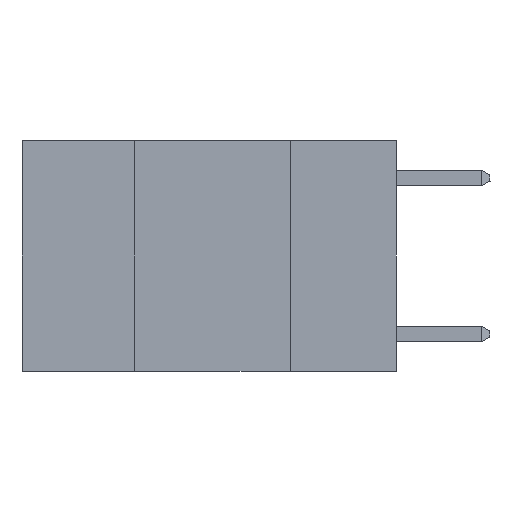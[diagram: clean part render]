
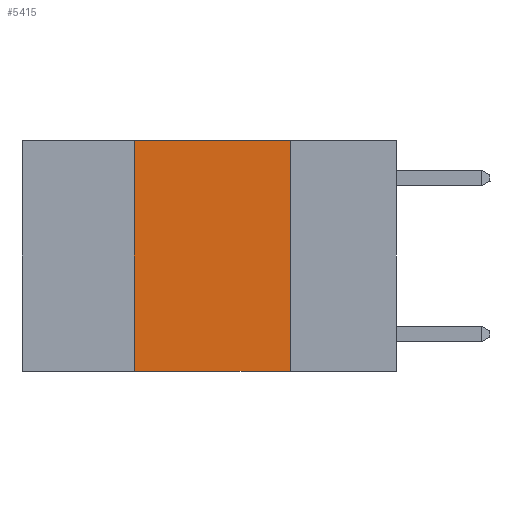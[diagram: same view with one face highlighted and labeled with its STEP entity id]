
A CAD part, left-side view. The second image highlights one B-rep face of the part: STEP entity #5415.
In plain terms, the highlighted planar face has unit normal (-1, 0, 0).
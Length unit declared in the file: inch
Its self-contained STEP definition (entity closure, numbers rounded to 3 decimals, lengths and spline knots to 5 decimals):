
#32 = VERTEX_POINT ( 'NONE', #3492 ) ;
#42 = CARTESIAN_POINT ( 'NONE',  ( 0., 0.17, -0.37 ) ) ;
#235 = VECTOR ( 'NONE', #409, 39.37008 ) ;
#409 = DIRECTION ( 'NONE',  ( 0., -1., 0. ) ) ;
#447 = DIRECTION ( 'NONE',  ( 0., 0., -1. ) ) ;
#834 = CARTESIAN_POINT ( 'NONE',  ( 0., 0.6, 0. ) ) ;
#1045 = VECTOR ( 'NONE', #3212, 39.37008 ) ;
#1571 = DIRECTION ( 'NONE',  ( 0., 0., -1. ) ) ;
#1638 = FACE_OUTER_BOUND ( 'NONE', #7906, .T. ) ;
#1929 = VECTOR ( 'NONE', #447, 39.37008 ) ;
#2073 = EDGE_CURVE ( 'NONE', #32, #7434, #4094, .T. ) ;
#2083 = ORIENTED_EDGE ( 'NONE', *, *, #8897, .T. ) ;
#2264 = AXIS2_PLACEMENT_3D ( 'NONE', #834, #6049, #1571 ) ;
#2320 = VERTEX_POINT ( 'NONE', #5282 ) ;
#2329 = CARTESIAN_POINT ( 'NONE',  ( 0., 0.42, 0. ) ) ;
#2740 = ORIENTED_EDGE ( 'NONE', *, *, #4214, .F. ) ;
#3212 = DIRECTION ( 'NONE',  ( 0., 0., 1. ) ) ;
#3402 = ORIENTED_EDGE ( 'NONE', *, *, #2073, .F. ) ;
#3492 = CARTESIAN_POINT ( 'NONE',  ( 0., 0.17, 0. ) ) ;
#4094 = LINE ( 'NONE', #5994, #1929 ) ;
#4214 = EDGE_CURVE ( 'NONE', #7386, #32, #8233, .T. ) ;
#4279 = CARTESIAN_POINT ( 'NONE',  ( 0., 0.6, 0. ) ) ;
#5282 = CARTESIAN_POINT ( 'NONE',  ( 0., 0.42, -0.37 ) ) ;
#5415 = ADVANCED_FACE ( 'NONE', ( #1638 ), #9289, .F. ) ;
#5878 = DIRECTION ( 'NONE',  ( 0., -1., 0. ) ) ;
#5994 = CARTESIAN_POINT ( 'NONE',  ( 0., 0.17, 0. ) ) ;
#6049 = DIRECTION ( 'NONE',  ( 1., 0., 0. ) ) ;
#6758 = CARTESIAN_POINT ( 'NONE',  ( 0., 0.42, 0. ) ) ;
#7359 = LINE ( 'NONE', #7895, #8665 ) ;
#7386 = VERTEX_POINT ( 'NONE', #6758 ) ;
#7434 = VERTEX_POINT ( 'NONE', #42 ) ;
#7473 = EDGE_CURVE ( 'NONE', #2320, #7386, #8688, .T. ) ;
#7895 = CARTESIAN_POINT ( 'NONE',  ( 0., 0.6, -0.37 ) ) ;
#7906 = EDGE_LOOP ( 'NONE', ( #3402, #2740, #8760, #2083 ) ) ;
#8233 = LINE ( 'NONE', #4279, #235 ) ;
#8665 = VECTOR ( 'NONE', #5878, 39.37008 ) ;
#8688 = LINE ( 'NONE', #2329, #1045 ) ;
#8760 = ORIENTED_EDGE ( 'NONE', *, *, #7473, .F. ) ;
#8897 = EDGE_CURVE ( 'NONE', #2320, #7434, #7359, .T. ) ;
#9289 = PLANE ( 'NONE',  #2264 ) ;
